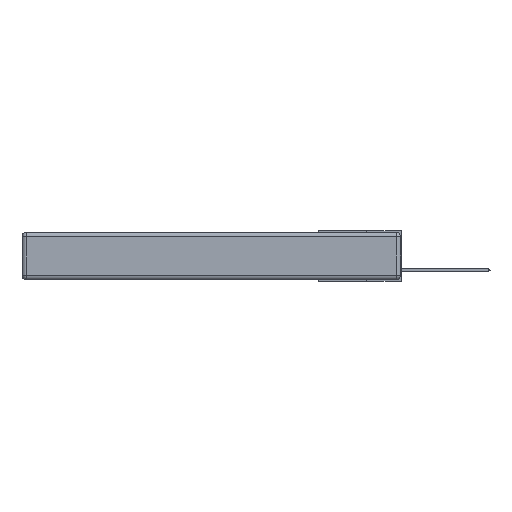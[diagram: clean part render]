
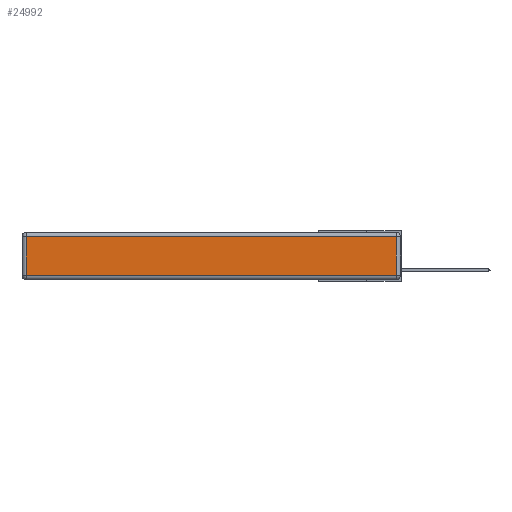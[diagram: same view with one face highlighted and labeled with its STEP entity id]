
A CAD part, left-side view. The second image highlights one B-rep face of the part: STEP entity #24992.
In plain terms, the highlighted planar face has unit normal (-1, 0, 0).
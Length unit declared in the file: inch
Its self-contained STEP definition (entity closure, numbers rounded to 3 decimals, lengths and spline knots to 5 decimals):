
#77 = CARTESIAN_POINT ( 'NONE',  ( 0., 0.03, -0.343 ) ) ;
#1708 = CARTESIAN_POINT ( 'NONE',  ( 0., 2.72, -0.343 ) ) ;
#2203 = VECTOR ( 'NONE', #4841, 39.37008 ) ;
#3432 = EDGE_CURVE ( 'NONE', #18228, #5847, #23314, .T. ) ;
#3816 = LINE ( 'NONE', #77, #2203 ) ;
#4841 = DIRECTION ( 'NONE',  ( 0., 0., 1. ) ) ;
#4939 = DIRECTION ( 'NONE',  ( -1., 0., 0. ) ) ;
#5148 = CARTESIAN_POINT ( 'NONE',  ( 0., 0., -0.343 ) ) ;
#5227 = FACE_OUTER_BOUND ( 'NONE', #17783, .T. ) ;
#5621 = ORIENTED_EDGE ( 'NONE', *, *, #32656, .T. ) ;
#5847 = VERTEX_POINT ( 'NONE', #18849 ) ;
#6368 = EDGE_CURVE ( 'NONE', #29874, #7560, #3816, .T. ) ;
#6949 = CARTESIAN_POINT ( 'NONE',  ( 0., 2.75, -0.03 ) ) ;
#7121 = VECTOR ( 'NONE', #29382, 39.37008 ) ;
#7162 = LINE ( 'NONE', #6949, #22152 ) ;
#7560 = VERTEX_POINT ( 'NONE', #26033 ) ;
#9210 = VECTOR ( 'NONE', #16825, 39.37008 ) ;
#9916 = PLANE ( 'NONE',  #30419 ) ;
#14063 = EDGE_CURVE ( 'NONE', #5847, #29874, #18278, .T. ) ;
#16019 = CARTESIAN_POINT ( 'NONE',  ( 0., 0.03, -0.313 ) ) ;
#16825 = DIRECTION ( 'NONE',  ( 0., -1., 0. ) ) ;
#17783 = EDGE_LOOP ( 'NONE', ( #27199, #31524, #5621, #32675 ) ) ;
#18228 = VERTEX_POINT ( 'NONE', #18529 ) ;
#18278 = LINE ( 'NONE', #29471, #9210 ) ;
#18529 = CARTESIAN_POINT ( 'NONE',  ( 0., 2.72, -0.03 ) ) ;
#18849 = CARTESIAN_POINT ( 'NONE',  ( 0., 2.72, -0.313 ) ) ;
#19223 = DIRECTION ( 'NONE',  ( 0., 1., 0. ) ) ;
#22152 = VECTOR ( 'NONE', #19223, 39.37008 ) ;
#23314 = LINE ( 'NONE', #1708, #7121 ) ;
#24992 = ADVANCED_FACE ( 'NONE', ( #5227 ), #9916, .T. ) ;
#26033 = CARTESIAN_POINT ( 'NONE',  ( 0., 0.03, -0.03 ) ) ;
#27199 = ORIENTED_EDGE ( 'NONE', *, *, #14063, .T. ) ;
#29382 = DIRECTION ( 'NONE',  ( 0., 0., -1. ) ) ;
#29471 = CARTESIAN_POINT ( 'NONE',  ( 0., 0., -0.313 ) ) ;
#29874 = VERTEX_POINT ( 'NONE', #16019 ) ;
#30419 = AXIS2_PLACEMENT_3D ( 'NONE', #5148, #4939, #30713 ) ;
#30713 = DIRECTION ( 'NONE',  ( 0., 0., 1. ) ) ;
#31524 = ORIENTED_EDGE ( 'NONE', *, *, #6368, .T. ) ;
#32656 = EDGE_CURVE ( 'NONE', #7560, #18228, #7162, .T. ) ;
#32675 = ORIENTED_EDGE ( 'NONE', *, *, #3432, .T. ) ;
